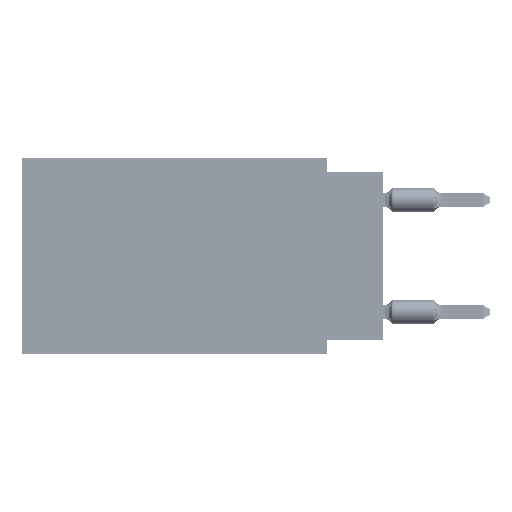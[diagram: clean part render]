
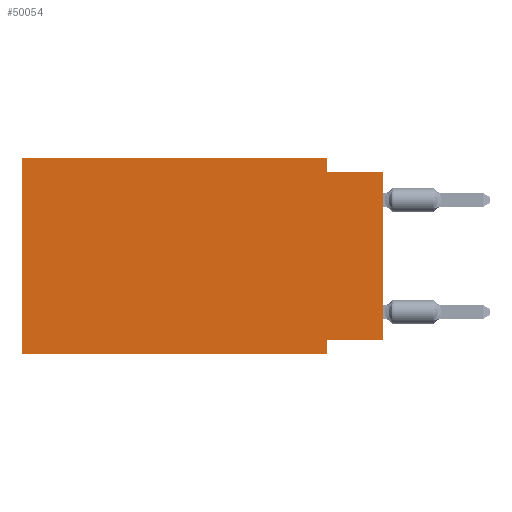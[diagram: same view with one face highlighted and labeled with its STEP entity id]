
A CAD part, left-side view. The second image highlights one B-rep face of the part: STEP entity #50054.
In plain terms, the highlighted planar face has unit normal (-1, 0, 0).
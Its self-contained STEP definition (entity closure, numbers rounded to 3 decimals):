
#2386 = EDGE_CURVE ( 'NONE', #6044, #112319, #62803, .T. ) ;
#2697 = CARTESIAN_POINT ( 'NONE',  ( 0., 2.54, -8.89 ) ) ;
#4294 = EDGE_CURVE ( 'NONE', #71855, #22581, #72313, .T. ) ;
#4830 = VECTOR ( 'NONE', #45498, 1000. ) ;
#5665 = FACE_OUTER_BOUND ( 'NONE', #85035, .T. ) ;
#5892 = ORIENTED_EDGE ( 'NONE', *, *, #89994, .F. ) ;
#6044 = VERTEX_POINT ( 'NONE', #55185 ) ;
#8110 = LINE ( 'NONE', #93714, #49066 ) ;
#10322 = DIRECTION ( 'NONE',  ( 0., 0., 1. ) ) ;
#17475 = VERTEX_POINT ( 'NONE', #87531 ) ;
#19094 = VERTEX_POINT ( 'NONE', #103017 ) ;
#20871 = AXIS2_PLACEMENT_3D ( 'NONE', #30808, #39906, #66704 ) ;
#21166 = ORIENTED_EDGE ( 'NONE', *, *, #4294, .F. ) ;
#22581 = VERTEX_POINT ( 'NONE', #81022 ) ;
#25640 = CARTESIAN_POINT ( 'NONE',  ( 0., 2.54, 0. ) ) ;
#30808 = CARTESIAN_POINT ( 'NONE',  ( 0., 16.383, 0. ) ) ;
#32535 = EDGE_CURVE ( 'NONE', #69463, #19094, #66541, .T. ) ;
#35057 = ORIENTED_EDGE ( 'NONE', *, *, #71224, .T. ) ;
#36538 = VECTOR ( 'NONE', #74299, 1000. ) ;
#37793 = LINE ( 'NONE', #56576, #36538 ) ;
#39906 = DIRECTION ( 'NONE',  ( 1., 0., 0. ) ) ;
#40720 = ORIENTED_EDGE ( 'NONE', *, *, #105811, .F. ) ;
#42754 = ORIENTED_EDGE ( 'NONE', *, *, #32535, .F. ) ;
#43300 = DIRECTION ( 'NONE',  ( 0., 0., -1. ) ) ;
#45004 = CARTESIAN_POINT ( 'NONE',  ( 0., 2.54, -8.255 ) ) ;
#45498 = DIRECTION ( 'NONE',  ( 0., 0., -1. ) ) ;
#49066 = VECTOR ( 'NONE', #78292, 1000. ) ;
#50054 = ADVANCED_FACE ( 'NONE', ( #5665 ), #110057, .F. ) ;
#55185 = CARTESIAN_POINT ( 'NONE',  ( 0., 0., -8.255 ) ) ;
#56576 = CARTESIAN_POINT ( 'NONE',  ( 0., 0., -0.635 ) ) ;
#59459 = LINE ( 'NONE', #61147, #67384 ) ;
#59665 = CARTESIAN_POINT ( 'NONE',  ( 0., 16.383, 0. ) ) ;
#59780 = ORIENTED_EDGE ( 'NONE', *, *, #85196, .F. ) ;
#60591 = LINE ( 'NONE', #77744, #108313 ) ;
#60858 = ORIENTED_EDGE ( 'NONE', *, *, #101961, .F. ) ;
#61147 = CARTESIAN_POINT ( 'NONE',  ( 0., 16.383, 0. ) ) ;
#61861 = VECTOR ( 'NONE', #43300, 1000. ) ;
#62234 = CARTESIAN_POINT ( 'NONE',  ( 0., 0., 0. ) ) ;
#62803 = LINE ( 'NONE', #62234, #90292 ) ;
#66541 = LINE ( 'NONE', #59665, #91930 ) ;
#66704 = DIRECTION ( 'NONE',  ( 0., 0., -1. ) ) ;
#67028 = CARTESIAN_POINT ( 'NONE',  ( 0., 16.383, -8.89 ) ) ;
#67384 = VECTOR ( 'NONE', #112524, 1000. ) ;
#69463 = VERTEX_POINT ( 'NONE', #67028 ) ;
#71224 = EDGE_CURVE ( 'NONE', #69463, #22581, #8110, .T. ) ;
#71447 = CARTESIAN_POINT ( 'NONE',  ( 0., 2.54, 0. ) ) ;
#71855 = VERTEX_POINT ( 'NONE', #45004 ) ;
#72313 = LINE ( 'NONE', #2697, #4830 ) ;
#74299 = DIRECTION ( 'NONE',  ( 0., -1., 0. ) ) ;
#76501 = ORIENTED_EDGE ( 'NONE', *, *, #2386, .T. ) ;
#77744 = CARTESIAN_POINT ( 'NONE',  ( 0., 0., -8.255 ) ) ;
#78292 = DIRECTION ( 'NONE',  ( 0., -1., 0. ) ) ;
#79231 = LINE ( 'NONE', #25640, #61861 ) ;
#79412 = DIRECTION ( 'NONE',  ( 0., 1., 0. ) ) ;
#81022 = CARTESIAN_POINT ( 'NONE',  ( 0., 2.54, -8.89 ) ) ;
#82757 = CARTESIAN_POINT ( 'NONE',  ( 0., 0., -0.635 ) ) ;
#85035 = EDGE_LOOP ( 'NONE', ( #76501, #5892, #60858, #40720, #42754, #35057, #21166, #59780 ) ) ;
#85196 = EDGE_CURVE ( 'NONE', #6044, #71855, #60591, .T. ) ;
#87531 = CARTESIAN_POINT ( 'NONE',  ( 0., 2.54, -0.635 ) ) ;
#88788 = VERTEX_POINT ( 'NONE', #71447 ) ;
#89994 = EDGE_CURVE ( 'NONE', #17475, #112319, #37793, .T. ) ;
#90292 = VECTOR ( 'NONE', #10322, 1000. ) ;
#91930 = VECTOR ( 'NONE', #92804, 1000. ) ;
#92804 = DIRECTION ( 'NONE',  ( 0., 0., 1. ) ) ;
#93714 = CARTESIAN_POINT ( 'NONE',  ( 0., 16.383, -8.89 ) ) ;
#101961 = EDGE_CURVE ( 'NONE', #88788, #17475, #79231, .T. ) ;
#103017 = CARTESIAN_POINT ( 'NONE',  ( 0., 16.383, 0. ) ) ;
#105811 = EDGE_CURVE ( 'NONE', #19094, #88788, #59459, .T. ) ;
#108313 = VECTOR ( 'NONE', #79412, 1000. ) ;
#110057 = PLANE ( 'NONE',  #20871 ) ;
#112319 = VERTEX_POINT ( 'NONE', #82757 ) ;
#112524 = DIRECTION ( 'NONE',  ( 0., -1., 0. ) ) ;
